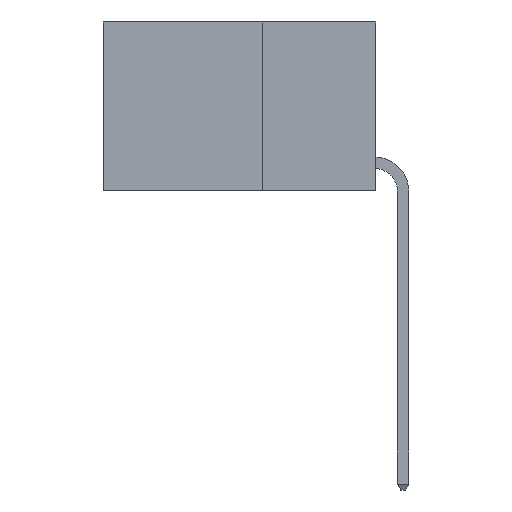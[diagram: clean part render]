
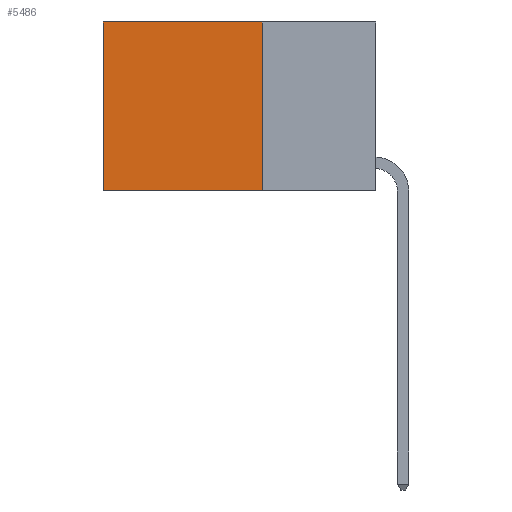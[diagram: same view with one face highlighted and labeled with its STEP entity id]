
A CAD part, left-side view. The second image highlights one B-rep face of the part: STEP entity #5486.
In plain terms, the highlighted planar face has unit normal (-1, 0, 0).
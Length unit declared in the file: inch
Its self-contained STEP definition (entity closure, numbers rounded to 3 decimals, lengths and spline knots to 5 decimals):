
#101 = DIRECTION ( 'NONE',  ( 0., 0., -1. ) ) ;
#360 = LINE ( 'NONE', #9783, #6047 ) ;
#435 = EDGE_CURVE ( 'NONE', #4017, #4556, #9689, .T. ) ;
#1362 = DIRECTION ( 'NONE',  ( 0., 0., -1. ) ) ;
#1512 = VECTOR ( 'NONE', #1362, 39.37008 ) ;
#1609 = CARTESIAN_POINT ( 'NONE',  ( 0.2625, 0.25, 0. ) ) ;
#1862 = CARTESIAN_POINT ( 'NONE',  ( 0.2625, 0.25, 0. ) ) ;
#1924 = EDGE_LOOP ( 'NONE', ( #9754, #9358, #10753, #5688 ) ) ;
#2637 = VERTEX_POINT ( 'NONE', #8167 ) ;
#4017 = VERTEX_POINT ( 'NONE', #8304 ) ;
#4053 = DIRECTION ( 'NONE',  ( 0., 0., -1. ) ) ;
#4191 = DIRECTION ( 'NONE',  ( 0., 1., 0. ) ) ;
#4556 = VERTEX_POINT ( 'NONE', #5716 ) ;
#5208 = EDGE_CURVE ( 'NONE', #6197, #4017, #360, .T. ) ;
#5249 = DIRECTION ( 'NONE',  ( 1., 0., 0. ) ) ;
#5486 = ADVANCED_FACE ( 'NONE', ( #7642 ), #10163, .F. ) ;
#5545 = CARTESIAN_POINT ( 'NONE',  ( 0.2625, 0.6, 0. ) ) ;
#5688 = ORIENTED_EDGE ( 'NONE', *, *, #7349, .T. ) ;
#5716 = CARTESIAN_POINT ( 'NONE',  ( 0.2625, 0.6, -0.37 ) ) ;
#6047 = VECTOR ( 'NONE', #4053, 39.37008 ) ;
#6197 = VERTEX_POINT ( 'NONE', #7737 ) ;
#6687 = VECTOR ( 'NONE', #4191, 39.37008 ) ;
#7349 = EDGE_CURVE ( 'NONE', #6197, #2637, #8863, .T. ) ;
#7642 = FACE_OUTER_BOUND ( 'NONE', #1924, .T. ) ;
#7737 = CARTESIAN_POINT ( 'NONE',  ( 0.2625, 0.25, 0. ) ) ;
#8167 = CARTESIAN_POINT ( 'NONE',  ( 0.2625, 0.6, 0. ) ) ;
#8304 = CARTESIAN_POINT ( 'NONE',  ( 0.2625, 0.25, -0.37 ) ) ;
#8863 = LINE ( 'NONE', #1609, #6687 ) ;
#9358 = ORIENTED_EDGE ( 'NONE', *, *, #435, .F. ) ;
#9548 = CARTESIAN_POINT ( 'NONE',  ( 0.2625, 0.25, -0.37 ) ) ;
#9647 = VECTOR ( 'NONE', #9687, 39.37008 ) ;
#9687 = DIRECTION ( 'NONE',  ( 0., 1., 0. ) ) ;
#9689 = LINE ( 'NONE', #9548, #9647 ) ;
#9754 = ORIENTED_EDGE ( 'NONE', *, *, #10531, .T. ) ;
#9783 = CARTESIAN_POINT ( 'NONE',  ( 0.2625, 0.25, 0. ) ) ;
#10059 = AXIS2_PLACEMENT_3D ( 'NONE', #1862, #5249, #101 ) ;
#10082 = LINE ( 'NONE', #5545, #1512 ) ;
#10163 = PLANE ( 'NONE',  #10059 ) ;
#10531 = EDGE_CURVE ( 'NONE', #2637, #4556, #10082, .T. ) ;
#10753 = ORIENTED_EDGE ( 'NONE', *, *, #5208, .F. ) ;
